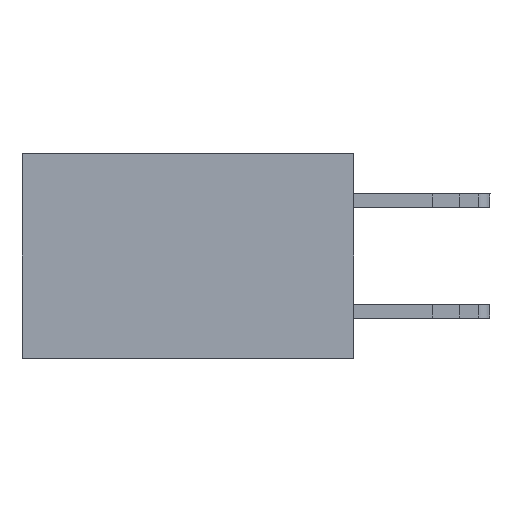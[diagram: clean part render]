
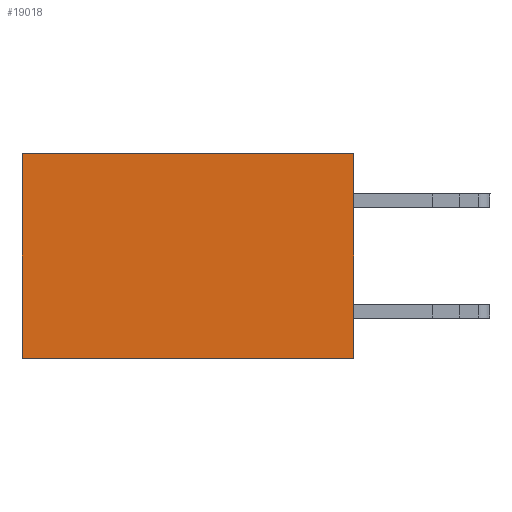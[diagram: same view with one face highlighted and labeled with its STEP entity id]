
A CAD part, left-side view. The second image highlights one B-rep face of the part: STEP entity #19018.
In plain terms, the highlighted planar face has unit normal (-1, 0, 0).
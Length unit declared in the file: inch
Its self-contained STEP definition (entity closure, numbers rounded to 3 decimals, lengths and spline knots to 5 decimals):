
#663 = EDGE_CURVE ( 'NONE', #7919, #13549, #5450, .T. ) ;
#963 = VERTEX_POINT ( 'NONE', #16869 ) ;
#1072 = VERTEX_POINT ( 'NONE', #4233 ) ;
#1435 = EDGE_CURVE ( 'NONE', #1072, #7919, #14223, .T. ) ;
#2048 = FACE_OUTER_BOUND ( 'NONE', #18344, .T. ) ;
#2054 = DIRECTION ( 'NONE',  ( 0., 1., 0. ) ) ;
#2971 = CARTESIAN_POINT ( 'NONE',  ( 0.2875, 0.6, -0.37 ) ) ;
#3072 = VECTOR ( 'NONE', #3912, 39.37008 ) ;
#3470 = VECTOR ( 'NONE', #2054, 39.37008 ) ;
#3565 = LINE ( 'NONE', #6994, #18531 ) ;
#3912 = DIRECTION ( 'NONE',  ( 0., 0., -1. ) ) ;
#4233 = CARTESIAN_POINT ( 'NONE',  ( 0.2875, 0., 0. ) ) ;
#5251 = LINE ( 'NONE', #12234, #3470 ) ;
#5450 = LINE ( 'NONE', #17398, #13118 ) ;
#5463 = ORIENTED_EDGE ( 'NONE', *, *, #663, .F. ) ;
#6994 = CARTESIAN_POINT ( 'NONE',  ( 0.2875, 0.6, 0. ) ) ;
#7919 = VERTEX_POINT ( 'NONE', #21838 ) ;
#9017 = CARTESIAN_POINT ( 'NONE',  ( 0.2875, 0., 0. ) ) ;
#9396 = DIRECTION ( 'NONE',  ( 0., 0., -1. ) ) ;
#9691 = ORIENTED_EDGE ( 'NONE', *, *, #21381, .T. ) ;
#9922 = ORIENTED_EDGE ( 'NONE', *, *, #1435, .F. ) ;
#12234 = CARTESIAN_POINT ( 'NONE',  ( 0.2875, 0., 0. ) ) ;
#12790 = CARTESIAN_POINT ( 'NONE',  ( 0.2875, 0., 0. ) ) ;
#13118 = VECTOR ( 'NONE', #21217, 39.37008 ) ;
#13549 = VERTEX_POINT ( 'NONE', #2971 ) ;
#13887 = DIRECTION ( 'NONE',  ( 0., 0., -1. ) ) ;
#14223 = LINE ( 'NONE', #9017, #3072 ) ;
#14250 = DIRECTION ( 'NONE',  ( 1., 0., 0. ) ) ;
#16869 = CARTESIAN_POINT ( 'NONE',  ( 0.2875, 0.6, 0. ) ) ;
#17398 = CARTESIAN_POINT ( 'NONE',  ( 0.2875, 0., -0.37 ) ) ;
#17734 = PLANE ( 'NONE',  #18515 ) ;
#18344 = EDGE_LOOP ( 'NONE', ( #19228, #5463, #9922, #9691 ) ) ;
#18515 = AXIS2_PLACEMENT_3D ( 'NONE', #12790, #14250, #9396 ) ;
#18531 = VECTOR ( 'NONE', #13887, 39.37008 ) ;
#19018 = ADVANCED_FACE ( 'NONE', ( #2048 ), #17734, .F. ) ;
#19228 = ORIENTED_EDGE ( 'NONE', *, *, #19367, .T. ) ;
#19367 = EDGE_CURVE ( 'NONE', #963, #13549, #3565, .T. ) ;
#21217 = DIRECTION ( 'NONE',  ( 0., 1., 0. ) ) ;
#21381 = EDGE_CURVE ( 'NONE', #1072, #963, #5251, .T. ) ;
#21838 = CARTESIAN_POINT ( 'NONE',  ( 0.2875, 0., -0.37 ) ) ;
